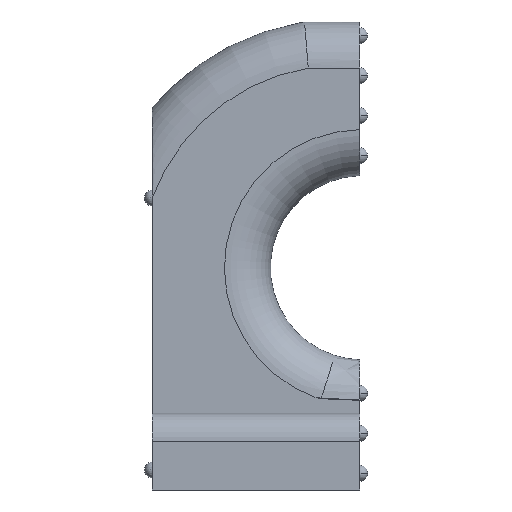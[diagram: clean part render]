
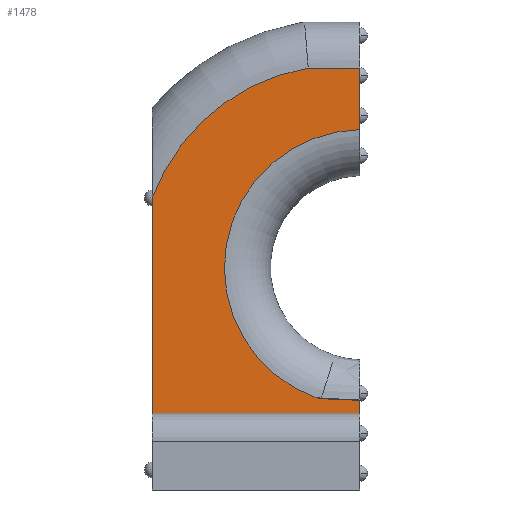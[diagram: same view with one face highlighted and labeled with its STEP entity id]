
A CAD part, front view. The second image highlights one B-rep face of the part: STEP entity #1478.
In plain terms, the highlighted planar face has unit normal (0, -1, 0).
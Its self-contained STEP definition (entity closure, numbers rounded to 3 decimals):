
#13 = AXIS2_PLACEMENT_3D ( 'NONE', #913, #911, #906 ) ;
#42 = AXIS2_PLACEMENT_3D ( 'NONE', #979, #978, #974 ) ;
#108 = CARTESIAN_POINT ( 'NONE',  ( -103.556, -36.842, -21.324 ) ) ;
#167 = CARTESIAN_POINT ( 'NONE',  ( -51.708, -36.842, -21.324 ) ) ;
#168 = CARTESIAN_POINT ( 'NONE',  ( -51.708, -36.842, -18.023 ) ) ;
#184 = CARTESIAN_POINT ( 'NONE',  ( -51.708, -36.842, 49.61 ) ) ;
#187 = CARTESIAN_POINT ( 'NONE',  ( -62.615, -36.842, -17.41 ) ) ;
#191 = CARTESIAN_POINT ( 'NONE',  ( -64.552, -36.842, 65.013 ) ) ;
#210 = EDGE_LOOP ( 'NONE', ( #989, #990, #514, #516, #519, #556, #577, #579, #580 ) ) ;
#411 = DIRECTION ( 'NONE',  ( 1., 0., 0. ) ) ;
#412 = DIRECTION ( 'NONE',  ( 0., 1., 0. ) ) ;
#418 = CARTESIAN_POINT ( 'NONE',  ( 168.194, -36.842, -34.139 ) ) ;
#431 = PLANE ( 'NONE',  #442 ) ;
#442 = AXIS2_PLACEMENT_3D ( 'NONE', #418, #412, #411 ) ;
#514 = ORIENTED_EDGE ( 'NONE', *, *, #1273, .T. ) ;
#516 = ORIENTED_EDGE ( 'NONE', *, *, #1085, .F. ) ;
#519 = ORIENTED_EDGE ( 'NONE', *, *, #1276, .F. ) ;
#539 = VERTEX_POINT ( 'NONE', #1883 ) ;
#556 = ORIENTED_EDGE ( 'NONE', *, *, #1281, .F. ) ;
#577 = ORIENTED_EDGE ( 'NONE', *, *, #1283, .T. ) ;
#579 = ORIENTED_EDGE ( 'NONE', *, *, #1013, .F. ) ;
#580 = ORIENTED_EDGE ( 'NONE', *, *, #1285, .T. ) ;
#805 = FACE_OUTER_BOUND ( 'NONE', #210, .T. ) ;
#880 = VECTOR ( 'NONE', #928, 1000. ) ;
#886 = CIRCLE ( 'NONE', #13, 34.52 ) ;
#893 = LINE ( 'NONE', #920, #880 ) ;
#894 = VECTOR ( 'NONE', #982, 1000. ) ;
#898 = LINE ( 'NONE', #970, #894 ) ;
#902 = CIRCLE ( 'NONE', #42, 50.644 ) ;
#906 = DIRECTION ( 'NONE',  ( 1., 0., 0. ) ) ;
#911 = DIRECTION ( 'NONE',  ( 0., 1., 0. ) ) ;
#913 = CARTESIAN_POINT ( 'NONE',  ( -50.998, -36.842, 15.097 ) ) ;
#920 = CARTESIAN_POINT ( 'NONE',  ( 103.318, -36.842, 65.013 ) ) ;
#922 = CARTESIAN_POINT ( 'NONE',  ( -61.29, -36.842, -17.645 ) ) ;
#923 = CARTESIAN_POINT ( 'NONE',  ( -61.732, -36.842, -17.571 ) ) ;
#926 = CARTESIAN_POINT ( 'NONE',  ( -62.615, -36.842, -17.41 ) ) ;
#928 = DIRECTION ( 'NONE',  ( -1., 0., 0. ) ) ;
#933 = CARTESIAN_POINT ( 'NONE',  ( -51.708, -36.842, -18.023 ) ) ;
#935 = CARTESIAN_POINT ( 'NONE',  ( -53.307, -36.842, -18.018 ) ) ;
#936 = CARTESIAN_POINT ( 'NONE',  ( -54.906, -36.842, -18.001 ) ) ;
#938 = CARTESIAN_POINT ( 'NONE',  ( -57.304, -36.842, -17.935 ) ) ;
#939 = CARTESIAN_POINT ( 'NONE',  ( -58.104, -36.842, -17.908 ) ) ;
#943 = CARTESIAN_POINT ( 'NONE',  ( -59.301, -36.842, -17.843 ) ) ;
#944 = CARTESIAN_POINT ( 'NONE',  ( -59.7, -36.842, -17.817 ) ) ;
#948 = CARTESIAN_POINT ( 'NONE',  ( -60.497, -36.842, -17.749 ) ) ;
#949 = CARTESIAN_POINT ( 'NONE',  ( -62.174, -36.842, -17.493 ) ) ;
#970 = CARTESIAN_POINT ( 'NONE',  ( -286.734, -36.842, -21.324 ) ) ;
#971 = CARTESIAN_POINT ( 'NONE',  ( -60.895, -36.842, -17.71 ) ) ;
#974 = DIRECTION ( 'NONE',  ( 1., 0., 0. ) ) ;
#978 = DIRECTION ( 'NONE',  ( 0., -1., 0. ) ) ;
#979 = CARTESIAN_POINT ( 'NONE',  ( -55.997, -36.842, 15.097 ) ) ;
#982 = DIRECTION ( 'NONE',  ( 1., 0., 0. ) ) ;
#989 = ORIENTED_EDGE ( 'NONE', *, *, #1262, .T. ) ;
#990 = ORIENTED_EDGE ( 'NONE', *, *, #1168, .T. ) ;
#994 = CARTESIAN_POINT ( 'NONE',  ( -61.29, -36.842, -17.645 ) ) ;
#1013 = EDGE_CURVE ( 'NONE', #539, #1655, #1106, .T. ) ;
#1017 = VERTEX_POINT ( 'NONE', #1570 ) ;
#1018 = VECTOR ( 'NONE', #1269, 1000. ) ;
#1048 = LINE ( 'NONE', #1274, #1018 ) ;
#1081 = VECTOR ( 'NONE', #1432, 1000. ) ;
#1085 = EDGE_CURVE ( 'NONE', #1687, #1670, #1095, .T. ) ;
#1095 = LINE ( 'NONE', #1349, #1081 ) ;
#1103 = VECTOR ( 'NONE', #1586, 1000. ) ;
#1106 = LINE ( 'NONE', #1581, #1103 ) ;
#1127 = B_SPLINE_CURVE_WITH_KNOTS ( 'NONE', 3,
 ( #994, #971, #948, #944, #943, #939, #938, #936, #935, #933 ),
 .UNSPECIFIED., .F., .F.,
 ( 4, 2, 2, 2, 4 ),
 ( 0., 0.001, 0.002, 0.005, 0.01 ),
 .UNSPECIFIED. ) ;
#1168 = EDGE_CURVE ( 'NONE', #1017, #1690, #1048, .T. ) ;
#1169 = VERTEX_POINT ( 'NONE', #1263 ) ;
#1262 = EDGE_CURVE ( 'NONE', #1679, #1017, #902, .T. ) ;
#1263 = CARTESIAN_POINT ( 'NONE',  ( -61.29, -36.842, -17.645 ) ) ;
#1269 = DIRECTION ( 'NONE',  ( 0., 0., -1. ) ) ;
#1273 = EDGE_CURVE ( 'NONE', #1690, #1670, #898, .T. ) ;
#1274 = CARTESIAN_POINT ( 'NONE',  ( -103.556, -36.842, -34.139 ) ) ;
#1276 = EDGE_CURVE ( 'NONE', #1169, #1687, #1127, .T. ) ;
#1281 = EDGE_CURVE ( 'NONE', #1651, #1169, #1330, .T. ) ;
#1283 = EDGE_CURVE ( 'NONE', #1651, #1655, #886, .T. ) ;
#1285 = EDGE_CURVE ( 'NONE', #539, #1679, #893, .T. ) ;
#1330 = B_SPLINE_CURVE_WITH_KNOTS ( 'NONE', 3,
 ( #926, #949, #923, #922 ),
 .UNSPECIFIED., .F., .F.,
 ( 4, 4 ),
 ( 0., 0.001 ),
 .UNSPECIFIED. ) ;
#1349 = CARTESIAN_POINT ( 'NONE',  ( -51.708, -36.842, -34.139 ) ) ;
#1432 = DIRECTION ( 'NONE',  ( 0., 0., -1. ) ) ;
#1478 = ADVANCED_FACE ( 'NONE', ( #805 ), #431, .F. ) ;
#1570 = CARTESIAN_POINT ( 'NONE',  ( -103.556, -36.842, 32.504 ) ) ;
#1581 = CARTESIAN_POINT ( 'NONE',  ( -51.708, -36.842, -34.139 ) ) ;
#1586 = DIRECTION ( 'NONE',  ( 0., 0., -1. ) ) ;
#1651 = VERTEX_POINT ( 'NONE', #187 ) ;
#1655 = VERTEX_POINT ( 'NONE', #184 ) ;
#1670 = VERTEX_POINT ( 'NONE', #167 ) ;
#1679 = VERTEX_POINT ( 'NONE', #191 ) ;
#1687 = VERTEX_POINT ( 'NONE', #168 ) ;
#1690 = VERTEX_POINT ( 'NONE', #108 ) ;
#1883 = CARTESIAN_POINT ( 'NONE',  ( -51.708, -36.842, 65.013 ) ) ;
